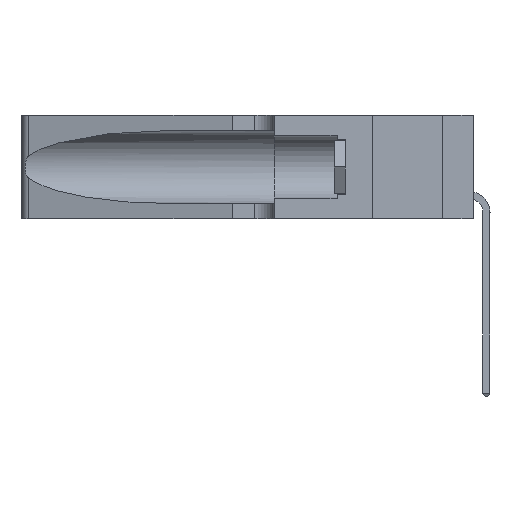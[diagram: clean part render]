
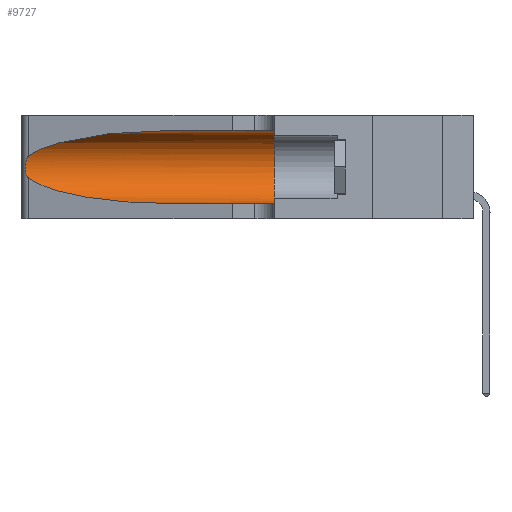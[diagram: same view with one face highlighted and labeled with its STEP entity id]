
A CAD part, left-side view. The second image highlights one B-rep face of the part: STEP entity #9727.
In plain terms, the highlighted cylindrical face has radius 3.308 mm (diameter 6.617 mm), a partial arc.
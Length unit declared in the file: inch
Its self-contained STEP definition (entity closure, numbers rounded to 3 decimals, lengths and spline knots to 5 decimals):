
#147 = ORIENTED_EDGE ( 'NONE', *, *, #10161, .T. ) ;
#359 = LINE ( 'NONE', #26429, #8938 ) ;
#861 = CARTESIAN_POINT ( 'NONE',  ( 0.1305, 0.35, 0.05475 ) ) ;
#1286 =( BOUNDED_CURVE ( )  B_SPLINE_CURVE ( 3, ( #1341, #3920, #23622, #6512 ),
 .UNSPECIFIED., .F., .T. ) 
 B_SPLINE_CURVE_WITH_KNOTS ( ( 4, 4 ),
 ( 1.5708, 2.84003 ),
 .UNSPECIFIED. ) 
 CURVE ( )  GEOMETRIC_REPRESENTATION_ITEM ( )  RATIONAL_B_SPLINE_CURVE ( ( 1., 0.87, 0.87, 1. ) ) 
 REPRESENTATION_ITEM ( '' )  );
#1341 = CARTESIAN_POINT ( 'NONE',  ( 0.1305, 0.72297, 0.31525 ) ) ;
#2454 = CARTESIAN_POINT ( 'NONE',  ( 0.2373, 1.15595, 0.08982 ) ) ;
#2465 = EDGE_CURVE ( 'NONE', #23871, #10902, #22567, .T. ) ;
#2832 = CARTESIAN_POINT ( 'NONE',  ( 0.1305, 0.72297, 0.31525 ) ) ;
#3006 = DIRECTION ( 'NONE',  ( 0., 0., 1. ) ) ;
#3920 = CARTESIAN_POINT ( 'NONE',  ( 0.18966, 0.96281, 0.31525 ) ) ;
#4022 = ORIENTED_EDGE ( 'NONE', *, *, #30800, .F. ) ;
#4031 = AXIS2_PLACEMENT_3D ( 'NONE', #23104, #13556, #3006 ) ;
#4445 = ORIENTED_EDGE ( 'NONE', *, *, #18392, .T. ) ;
#4845 = CARTESIAN_POINT ( 'NONE',  ( 0.18966, 0.96281, 0.05475 ) ) ;
#5104 = VERTEX_POINT ( 'NONE', #8859 ) ;
#5199 = VERTEX_POINT ( 'NONE', #11057 ) ;
#5487 = LINE ( 'NONE', #13152, #16344 ) ;
#5933 = ORIENTED_EDGE ( 'NONE', *, *, #21027, .T. ) ;
#6512 = CARTESIAN_POINT ( 'NONE',  ( 0.25487, 1.22718, 0.22369 ) ) ;
#6779 = B_SPLINE_CURVE_WITH_KNOTS ( 'NONE', 3,
 ( #9407, #16307, #30904, #23592, #9312, #26103, #30806, #11718, #18904, #16619, #16520, #29155, #21830, #26726 ),
 .UNSPECIFIED., .F., .F.,
 ( 4, 2, 2, 2, 2, 2, 4 ),
 ( 0., 0.00027, 0.00053, 0.00107, 0.0016, 0.00187, 0.00214 ),
 .UNSPECIFIED. ) ;
#6873 = VERTEX_POINT ( 'NONE', #2832 ) ;
#7232 = CARTESIAN_POINT ( 'NONE',  ( 0.1305, 0.35, 0.31525 ) ) ;
#8130 =( BOUNDED_CURVE ( )  B_SPLINE_CURVE ( 3, ( #28775, #2454, #4845, #16764 ),
 .UNSPECIFIED., .F., .F. ) 
 B_SPLINE_CURVE_WITH_KNOTS ( ( 4, 4 ),
 ( 3.44316, 4.71239 ),
 .UNSPECIFIED. ) 
 CURVE ( )  GEOMETRIC_REPRESENTATION_ITEM ( )  RATIONAL_B_SPLINE_CURVE ( ( 1., 0.87, 0.87, 1. ) ) 
 REPRESENTATION_ITEM ( '' )  );
#8859 = CARTESIAN_POINT ( 'NONE',  ( 0.25487, 1.22718, 0.14631 ) ) ;
#8938 = VECTOR ( 'NONE', #21953, 39.37008 ) ;
#9312 = CARTESIAN_POINT ( 'NONE',  ( 0.25854, 1.2359, 0.20912 ) ) ;
#9407 = CARTESIAN_POINT ( 'NONE',  ( 0.25487, 1.22718, 0.22369 ) ) ;
#9727 = ADVANCED_FACE ( 'NONE', ( #16092 ), #27299, .F. ) ;
#10161 = EDGE_CURVE ( 'NONE', #11946, #10902, #359, .T. ) ;
#10730 = DIRECTION ( 'NONE',  ( 0., -1., 0. ) ) ;
#10902 = VERTEX_POINT ( 'NONE', #861 ) ;
#10921 = CARTESIAN_POINT ( 'NONE',  ( 0.1305, 1.61858, 0.185 ) ) ;
#11057 = CARTESIAN_POINT ( 'NONE',  ( 0.25487, 1.22718, 0.22369 ) ) ;
#11718 = CARTESIAN_POINT ( 'NONE',  ( 0.26075, 1.23896, 0.178 ) ) ;
#11946 = VERTEX_POINT ( 'NONE', #21339 ) ;
#13047 = ORIENTED_EDGE ( 'NONE', *, *, #28592, .T. ) ;
#13152 = CARTESIAN_POINT ( 'NONE',  ( 0.1305, 1.61858, 0.31525 ) ) ;
#13556 = DIRECTION ( 'NONE',  ( 0., 1., 0. ) ) ;
#15599 = DIRECTION ( 'NONE',  ( 0., 0., -1. ) ) ;
#16092 = FACE_OUTER_BOUND ( 'NONE', #25752, .T. ) ;
#16307 = CARTESIAN_POINT ( 'NONE',  ( 0.25555, 1.22994, 0.2215 ) ) ;
#16344 = VECTOR ( 'NONE', #10730, 39.37008 ) ;
#16520 = CARTESIAN_POINT ( 'NONE',  ( 0.25789, 1.23486, 0.15765 ) ) ;
#16619 = CARTESIAN_POINT ( 'NONE',  ( 0.25856, 1.23593, 0.16098 ) ) ;
#16764 = CARTESIAN_POINT ( 'NONE',  ( 0.1305, 0.72297, 0.05475 ) ) ;
#17862 = ORIENTED_EDGE ( 'NONE', *, *, #2465, .F. ) ;
#18392 = EDGE_CURVE ( 'NONE', #5199, #5104, #6779, .T. ) ;
#18904 = CARTESIAN_POINT ( 'NONE',  ( 0.26017, 1.23833, 0.17102 ) ) ;
#21027 = EDGE_CURVE ( 'NONE', #5104, #11946, #8130, .T. ) ;
#21339 = CARTESIAN_POINT ( 'NONE',  ( 0.1305, 0.72297, 0.05475 ) ) ;
#21359 = AXIS2_PLACEMENT_3D ( 'NONE', #10921, #27408, #15599 ) ;
#21830 = CARTESIAN_POINT ( 'NONE',  ( 0.25555, 1.22993, 0.14849 ) ) ;
#21953 = DIRECTION ( 'NONE',  ( 0., -1., 0. ) ) ;
#22567 = CIRCLE ( 'NONE', #4031, 0.13025 ) ;
#23104 = CARTESIAN_POINT ( 'NONE',  ( 0.1305, 0.35, 0.185 ) ) ;
#23592 = CARTESIAN_POINT ( 'NONE',  ( 0.25787, 1.23484, 0.2124 ) ) ;
#23622 = CARTESIAN_POINT ( 'NONE',  ( 0.2373, 1.15595, 0.28018 ) ) ;
#23871 = VERTEX_POINT ( 'NONE', #7232 ) ;
#25752 = EDGE_LOOP ( 'NONE', ( #13047, #4445, #5933, #147, #17862, #4022 ) ) ;
#26103 = CARTESIAN_POINT ( 'NONE',  ( 0.26018, 1.23835, 0.19895 ) ) ;
#26429 = CARTESIAN_POINT ( 'NONE',  ( 0.1305, 1.61858, 0.05475 ) ) ;
#26726 = CARTESIAN_POINT ( 'NONE',  ( 0.25487, 1.22718, 0.14631 ) ) ;
#27299 = CYLINDRICAL_SURFACE ( 'NONE', #21359, 0.13025 ) ;
#27408 = DIRECTION ( 'NONE',  ( 0., -1., 0. ) ) ;
#28592 = EDGE_CURVE ( 'NONE', #6873, #5199, #1286, .T. ) ;
#28775 = CARTESIAN_POINT ( 'NONE',  ( 0.25487, 1.22718, 0.14631 ) ) ;
#29155 = CARTESIAN_POINT ( 'NONE',  ( 0.25639, 1.23186, 0.15144 ) ) ;
#30800 = EDGE_CURVE ( 'NONE', #6873, #23871, #5487, .T. ) ;
#30806 = CARTESIAN_POINT ( 'NONE',  ( 0.26075, 1.23896, 0.19203 ) ) ;
#30904 = CARTESIAN_POINT ( 'NONE',  ( 0.25639, 1.23184, 0.21858 ) ) ;
